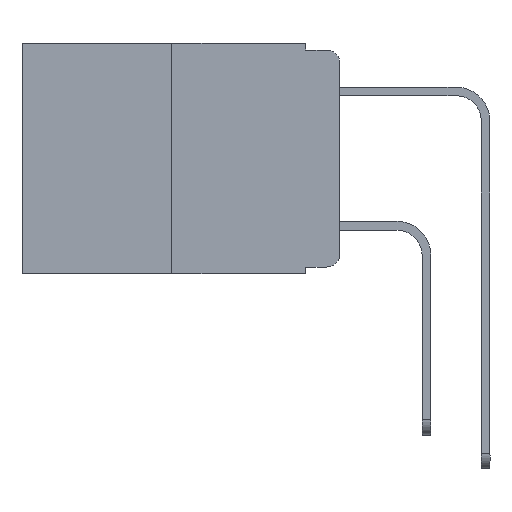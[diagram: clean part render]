
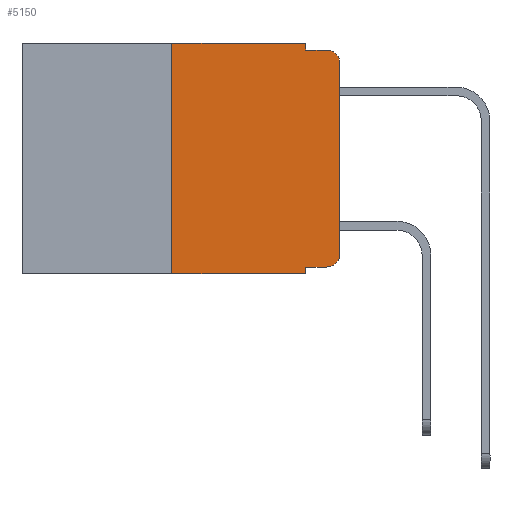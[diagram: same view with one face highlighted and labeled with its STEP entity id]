
A CAD part, left-side view. The second image highlights one B-rep face of the part: STEP entity #5150.
In plain terms, the highlighted planar face has unit normal (-1, 0, 0).
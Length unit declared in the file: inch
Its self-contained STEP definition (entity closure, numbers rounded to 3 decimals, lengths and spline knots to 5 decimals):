
#102 = ORIENTED_EDGE ( 'NONE', *, *, #3110, .T. ) ;
#129 = DIRECTION ( 'NONE',  ( 0., -1., 0. ) ) ;
#246 = VERTEX_POINT ( 'NONE', #1933 ) ;
#727 = VECTOR ( 'NONE', #2204, 39.37008 ) ;
#807 = VECTOR ( 'NONE', #9330, 39.37008 ) ;
#819 = CARTESIAN_POINT ( 'NONE',  ( 0., 0.02, -0.313 ) ) ;
#900 = CARTESIAN_POINT ( 'NONE',  ( 0., 0.473, 0. ) ) ;
#959 = CARTESIAN_POINT ( 'NONE',  ( 0., 0.25, 0. ) ) ;
#1041 = DIRECTION ( 'NONE',  ( 0., 0., 1. ) ) ;
#1100 = CIRCLE ( 'NONE', #8552, 0.02 ) ;
#1537 = DIRECTION ( 'NONE',  ( 0., 0., -1. ) ) ;
#1554 = CIRCLE ( 'NONE', #10656, 0.02 ) ;
#1779 = CARTESIAN_POINT ( 'NONE',  ( 0., 0.25, 0. ) ) ;
#1888 = DIRECTION ( 'NONE',  ( -1., 0., 0. ) ) ;
#1933 = CARTESIAN_POINT ( 'NONE',  ( 0., 0.25, -0.343 ) ) ;
#2204 = DIRECTION ( 'NONE',  ( 0., -1., 0. ) ) ;
#2602 = DIRECTION ( 'NONE',  ( 0., 0., -1. ) ) ;
#2637 = CARTESIAN_POINT ( 'NONE',  ( 0., 0.02, -0.01 ) ) ;
#2806 = VERTEX_POINT ( 'NONE', #2637 ) ;
#2946 = LINE ( 'NONE', #3961, #9846 ) ;
#2987 = ORIENTED_EDGE ( 'NONE', *, *, #7194, .T. ) ;
#3084 = CARTESIAN_POINT ( 'NONE',  ( 0., 0.051, -0.343 ) ) ;
#3109 = LINE ( 'NONE', #10064, #807 ) ;
#3110 = EDGE_CURVE ( 'NONE', #3385, #2806, #1554, .T. ) ;
#3260 = CARTESIAN_POINT ( 'NONE',  ( 0., 0.051, -0.333 ) ) ;
#3385 = VERTEX_POINT ( 'NONE', #7623 ) ;
#3537 = LINE ( 'NONE', #1779, #3975 ) ;
#3666 = VERTEX_POINT ( 'NONE', #959 ) ;
#3851 = CARTESIAN_POINT ( 'NONE',  ( 0., 0.051, -0.01 ) ) ;
#3872 = EDGE_CURVE ( 'NONE', #9629, #5893, #3109, .T. ) ;
#3961 = CARTESIAN_POINT ( 'NONE',  ( 0., 0.473, 0. ) ) ;
#3975 = VECTOR ( 'NONE', #1041, 39.37008 ) ;
#5141 = LINE ( 'NONE', #5238, #8568 ) ;
#5150 = ADVANCED_FACE ( 'NONE', ( #5907 ), #10472, .F. ) ;
#5238 = CARTESIAN_POINT ( 'NONE',  ( 0., 0.051, -0.01 ) ) ;
#5599 = CARTESIAN_POINT ( 'NONE',  ( 0., 0.473, -0.343 ) ) ;
#5612 = EDGE_CURVE ( 'NONE', #246, #3666, #3537, .T. ) ;
#5869 = CARTESIAN_POINT ( 'NONE',  ( 0., 0.02, -0.03 ) ) ;
#5893 = VERTEX_POINT ( 'NONE', #3084 ) ;
#5907 = FACE_OUTER_BOUND ( 'NONE', #6634, .T. ) ;
#6151 = CARTESIAN_POINT ( 'NONE',  ( 0., 0.02, -0.333 ) ) ;
#6166 = VECTOR ( 'NONE', #10432, 39.37008 ) ;
#6634 = EDGE_LOOP ( 'NONE', ( #9936, #102, #8440, #9517, #8976, #10188, #2987, #7607, #10118, #8575 ) ) ;
#6666 = LINE ( 'NONE', #3260, #8902 ) ;
#6865 = AXIS2_PLACEMENT_3D ( 'NONE', #900, #8473, #2602 ) ;
#7037 = CARTESIAN_POINT ( 'NONE',  ( 0., 0., 0. ) ) ;
#7194 = EDGE_CURVE ( 'NONE', #246, #5893, #7391, .T. ) ;
#7220 = VERTEX_POINT ( 'NONE', #3851 ) ;
#7391 = LINE ( 'NONE', #5599, #727 ) ;
#7544 = LINE ( 'NONE', #9363, #10745 ) ;
#7607 = ORIENTED_EDGE ( 'NONE', *, *, #3872, .F. ) ;
#7623 = CARTESIAN_POINT ( 'NONE',  ( 0., 0., -0.03 ) ) ;
#7833 = EDGE_CURVE ( 'NONE', #9475, #3385, #10307, .T. ) ;
#8324 = DIRECTION ( 'NONE',  ( 0., 0., -1. ) ) ;
#8440 = ORIENTED_EDGE ( 'NONE', *, *, #8543, .F. ) ;
#8473 = DIRECTION ( 'NONE',  ( 1., 0., 0. ) ) ;
#8543 = EDGE_CURVE ( 'NONE', #7220, #2806, #5141, .T. ) ;
#8552 = AXIS2_PLACEMENT_3D ( 'NONE', #819, #1888, #10383 ) ;
#8568 = VECTOR ( 'NONE', #129, 39.37008 ) ;
#8575 = ORIENTED_EDGE ( 'NONE', *, *, #10985, .T. ) ;
#8675 = EDGE_CURVE ( 'NONE', #3666, #8963, #2946, .T. ) ;
#8902 = VECTOR ( 'NONE', #11019, 39.37008 ) ;
#8963 = VERTEX_POINT ( 'NONE', #10628 ) ;
#8976 = ORIENTED_EDGE ( 'NONE', *, *, #8675, .F. ) ;
#9330 = DIRECTION ( 'NONE',  ( 0., 0., -1. ) ) ;
#9353 = DIRECTION ( 'NONE',  ( -1., 0., 0. ) ) ;
#9363 = CARTESIAN_POINT ( 'NONE',  ( 0., 0.051, 0. ) ) ;
#9475 = VERTEX_POINT ( 'NONE', #10670 ) ;
#9517 = ORIENTED_EDGE ( 'NONE', *, *, #10893, .F. ) ;
#9629 = VERTEX_POINT ( 'NONE', #10958 ) ;
#9846 = VECTOR ( 'NONE', #9897, 39.37008 ) ;
#9897 = DIRECTION ( 'NONE',  ( 0., -1., 0. ) ) ;
#9936 = ORIENTED_EDGE ( 'NONE', *, *, #7833, .T. ) ;
#10064 = CARTESIAN_POINT ( 'NONE',  ( 0., 0.051, 0. ) ) ;
#10118 = ORIENTED_EDGE ( 'NONE', *, *, #10409, .T. ) ;
#10188 = ORIENTED_EDGE ( 'NONE', *, *, #5612, .F. ) ;
#10307 = LINE ( 'NONE', #7037, #6166 ) ;
#10383 = DIRECTION ( 'NONE',  ( 0., 0., -1. ) ) ;
#10409 = EDGE_CURVE ( 'NONE', #9629, #10586, #6666, .T. ) ;
#10432 = DIRECTION ( 'NONE',  ( 0., 0., 1. ) ) ;
#10472 = PLANE ( 'NONE',  #6865 ) ;
#10586 = VERTEX_POINT ( 'NONE', #6151 ) ;
#10628 = CARTESIAN_POINT ( 'NONE',  ( 0., 0.051, 0. ) ) ;
#10656 = AXIS2_PLACEMENT_3D ( 'NONE', #5869, #9353, #1537 ) ;
#10670 = CARTESIAN_POINT ( 'NONE',  ( 0., 0., -0.313 ) ) ;
#10745 = VECTOR ( 'NONE', #8324, 39.37008 ) ;
#10893 = EDGE_CURVE ( 'NONE', #8963, #7220, #7544, .T. ) ;
#10958 = CARTESIAN_POINT ( 'NONE',  ( 0., 0.051, -0.333 ) ) ;
#10985 = EDGE_CURVE ( 'NONE', #10586, #9475, #1100, .T. ) ;
#11019 = DIRECTION ( 'NONE',  ( 0., -1., 0. ) ) ;
